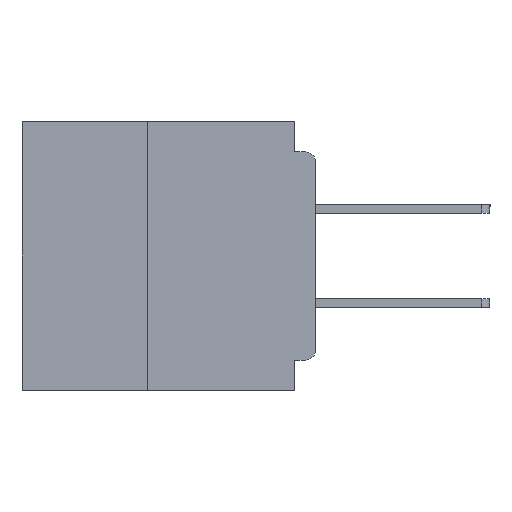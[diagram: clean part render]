
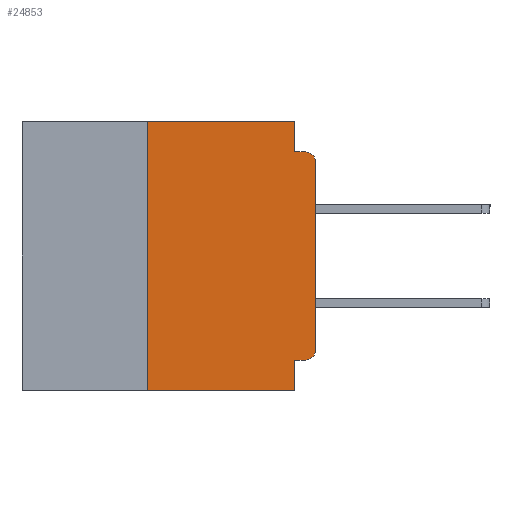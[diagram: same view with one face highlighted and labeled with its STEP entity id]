
A CAD part, left-side view. The second image highlights one B-rep face of the part: STEP entity #24853.
In plain terms, the highlighted planar face has unit normal (-1, 0, 0).
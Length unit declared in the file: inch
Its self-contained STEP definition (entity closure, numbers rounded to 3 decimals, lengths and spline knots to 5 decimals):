
#315 = LINE ( 'NONE', #21911, #38391 ) ;
#522 = VECTOR ( 'NONE', #48478, 39.37008 ) ;
#1276 = CARTESIAN_POINT ( 'NONE',  ( 0., 0., -0.34 ) ) ;
#1360 = ORIENTED_EDGE ( 'NONE', *, *, #44711, .F. ) ;
#4535 = VERTEX_POINT ( 'NONE', #38142 ) ;
#4848 = DIRECTION ( 'NONE',  ( 0., 0., -1. ) ) ;
#5576 = VECTOR ( 'NONE', #17892, 39.37008 ) ;
#5647 = EDGE_CURVE ( 'NONE', #46056, #13070, #30929, .T. ) ;
#6539 = CARTESIAN_POINT ( 'NONE',  ( 0., 0.015, -0.34 ) ) ;
#6789 = ORIENTED_EDGE ( 'NONE', *, *, #42313, .T. ) ;
#6930 = CARTESIAN_POINT ( 'NONE',  ( 0., 0.25, 0. ) ) ;
#7308 = EDGE_CURVE ( 'NONE', #43095, #28735, #47770, .T. ) ;
#7540 = VECTOR ( 'NONE', #4848, 39.37008 ) ;
#7999 = CIRCLE ( 'NONE', #42630, 0.015 ) ;
#8233 = CARTESIAN_POINT ( 'NONE',  ( 0., 0., 0. ) ) ;
#8711 = EDGE_CURVE ( 'NONE', #43363, #34901, #41777, .T. ) ;
#8826 = ORIENTED_EDGE ( 'NONE', *, *, #21793, .T. ) ;
#9764 = CARTESIAN_POINT ( 'NONE',  ( 0., 0.031, -0.355 ) ) ;
#10397 = DIRECTION ( 'NONE',  ( 0., 0., -1. ) ) ;
#10399 = DIRECTION ( 'NONE',  ( 0., -1., 0. ) ) ;
#10659 = DIRECTION ( 'NONE',  ( 0., 1., 0. ) ) ;
#12070 = DIRECTION ( 'NONE',  ( 0., 0., 1. ) ) ;
#12971 = CARTESIAN_POINT ( 'NONE',  ( 0., 0.031, -0.045 ) ) ;
#12998 = CARTESIAN_POINT ( 'NONE',  ( 0., 0.015, -0.06 ) ) ;
#13070 = VERTEX_POINT ( 'NONE', #28099 ) ;
#13907 = DIRECTION ( 'NONE',  ( 0., 0., 1. ) ) ;
#15120 = CIRCLE ( 'NONE', #46340, 0.015 ) ;
#16834 = DIRECTION ( 'NONE',  ( 0., 0., -1. ) ) ;
#17892 = DIRECTION ( 'NONE',  ( 0., -1., 0. ) ) ;
#18275 = ORIENTED_EDGE ( 'NONE', *, *, #31084, .F. ) ;
#19082 = CARTESIAN_POINT ( 'NONE',  ( 0., 0.031, 0. ) ) ;
#21619 = PLANE ( 'NONE',  #25221 ) ;
#21793 = EDGE_CURVE ( 'NONE', #4535, #24616, #7999, .T. ) ;
#21796 = EDGE_CURVE ( 'NONE', #34901, #23818, #35945, .T. ) ;
#21911 = CARTESIAN_POINT ( 'NONE',  ( 0., 0.437, -0.4 ) ) ;
#22860 = VERTEX_POINT ( 'NONE', #27781 ) ;
#23818 = VERTEX_POINT ( 'NONE', #19082 ) ;
#24616 = VERTEX_POINT ( 'NONE', #1276 ) ;
#24853 = ADVANCED_FACE ( 'NONE', ( #29084 ), #21619, .F. ) ;
#25221 = AXIS2_PLACEMENT_3D ( 'NONE', #36709, #47959, #25452 ) ;
#25452 = DIRECTION ( 'NONE',  ( 0., 0., -1. ) ) ;
#25804 = CARTESIAN_POINT ( 'NONE',  ( 0., 0.031, -0.4 ) ) ;
#26119 = ORIENTED_EDGE ( 'NONE', *, *, #21796, .F. ) ;
#27434 = VECTOR ( 'NONE', #10659, 39.37008 ) ;
#27707 = ORIENTED_EDGE ( 'NONE', *, *, #7308, .F. ) ;
#27781 = CARTESIAN_POINT ( 'NONE',  ( 0., 0., -0.06 ) ) ;
#28099 = CARTESIAN_POINT ( 'NONE',  ( 0., 0.015, -0.045 ) ) ;
#28735 = VERTEX_POINT ( 'NONE', #25804 ) ;
#29084 = FACE_OUTER_BOUND ( 'NONE', #38039, .T. ) ;
#29335 = CARTESIAN_POINT ( 'NONE',  ( 0., 0.437, 0. ) ) ;
#29770 = CARTESIAN_POINT ( 'NONE',  ( 0., 0., -0.045 ) ) ;
#29983 = ORIENTED_EDGE ( 'NONE', *, *, #36517, .T. ) ;
#30929 = LINE ( 'NONE', #29770, #522 ) ;
#31084 = EDGE_CURVE ( 'NONE', #4535, #43095, #37489, .T. ) ;
#31467 = CARTESIAN_POINT ( 'NONE',  ( 0., 0.031, -0.4 ) ) ;
#31881 = EDGE_CURVE ( 'NONE', #24616, #22860, #39722, .T. ) ;
#33160 = DIRECTION ( 'NONE',  ( -1., 0., 0. ) ) ;
#34460 = VECTOR ( 'NONE', #38979, 39.37008 ) ;
#34666 = CARTESIAN_POINT ( 'NONE',  ( 0., 0.25, -0.4 ) ) ;
#34901 = VERTEX_POINT ( 'NONE', #6930 ) ;
#35945 = LINE ( 'NONE', #29335, #5576 ) ;
#36467 = ORIENTED_EDGE ( 'NONE', *, *, #31881, .T. ) ;
#36502 = ORIENTED_EDGE ( 'NONE', *, *, #8711, .F. ) ;
#36517 = EDGE_CURVE ( 'NONE', #43363, #28735, #315, .T. ) ;
#36709 = CARTESIAN_POINT ( 'NONE',  ( 0., 0.437, 0. ) ) ;
#36817 = CARTESIAN_POINT ( 'NONE',  ( 0., 0.25, -0.4 ) ) ;
#37217 = CARTESIAN_POINT ( 'NONE',  ( 0., 0., -0.355 ) ) ;
#37489 = LINE ( 'NONE', #37217, #27434 ) ;
#38039 = EDGE_LOOP ( 'NONE', ( #36467, #6789, #44038, #1360, #26119, #36502, #29983, #27707, #18275, #8826 ) ) ;
#38142 = CARTESIAN_POINT ( 'NONE',  ( 0., 0.015, -0.355 ) ) ;
#38391 = VECTOR ( 'NONE', #10399, 39.37008 ) ;
#38567 = VECTOR ( 'NONE', #12070, 39.37008 ) ;
#38979 = DIRECTION ( 'NONE',  ( 0., 0., -1. ) ) ;
#39435 = VECTOR ( 'NONE', #13907, 39.37008 ) ;
#39519 = DIRECTION ( 'NONE',  ( -1., 0., 0. ) ) ;
#39722 = LINE ( 'NONE', #8233, #38567 ) ;
#41777 = LINE ( 'NONE', #36817, #39435 ) ;
#42313 = EDGE_CURVE ( 'NONE', #22860, #13070, #15120, .T. ) ;
#42579 = CARTESIAN_POINT ( 'NONE',  ( 0., 0.031, 0. ) ) ;
#42630 = AXIS2_PLACEMENT_3D ( 'NONE', #6539, #33160, #10397 ) ;
#43095 = VERTEX_POINT ( 'NONE', #9764 ) ;
#43363 = VERTEX_POINT ( 'NONE', #34666 ) ;
#44038 = ORIENTED_EDGE ( 'NONE', *, *, #5647, .F. ) ;
#44711 = EDGE_CURVE ( 'NONE', #23818, #46056, #45590, .T. ) ;
#45590 = LINE ( 'NONE', #42579, #34460 ) ;
#46056 = VERTEX_POINT ( 'NONE', #12971 ) ;
#46340 = AXIS2_PLACEMENT_3D ( 'NONE', #12998, #39519, #16834 ) ;
#47770 = LINE ( 'NONE', #31467, #7540 ) ;
#47959 = DIRECTION ( 'NONE',  ( 1., 0., 0. ) ) ;
#48478 = DIRECTION ( 'NONE',  ( 0., -1., 0. ) ) ;
